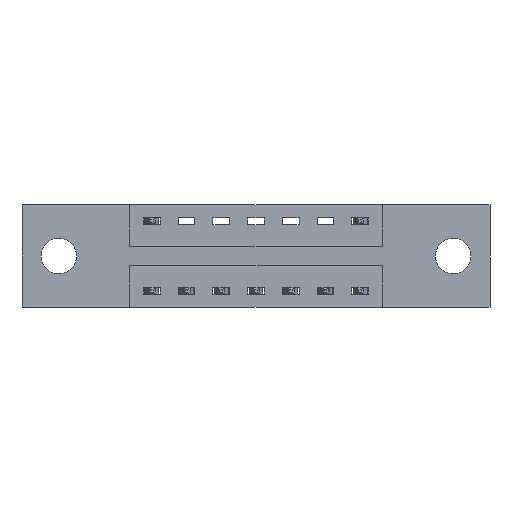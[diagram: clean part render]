
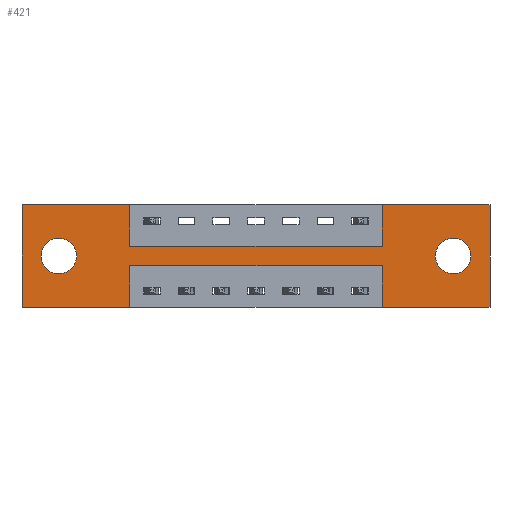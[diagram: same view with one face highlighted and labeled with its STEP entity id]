
A CAD part, front view. The second image highlights one B-rep face of the part: STEP entity #421.
In plain terms, the highlighted planar face has unit normal (0, -1, 0).
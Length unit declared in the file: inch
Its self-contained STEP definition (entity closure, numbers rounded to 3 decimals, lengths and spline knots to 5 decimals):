
#35 = DIRECTION ( 'NONE',  ( -1., 0., 0. ) ) ;
#144 = FACE_BOUND ( 'NONE', #7041, .T. ) ;
#194 = VERTEX_POINT ( 'NONE', #1288 ) ;
#335 = LINE ( 'NONE', #1972, #2369 ) ;
#369 = FACE_BOUND ( 'NONE', #668, .T. ) ;
#400 = CARTESIAN_POINT ( 'NONE',  ( 0.3875, 0., 0. ) ) ;
#421 = ADVANCED_FACE ( 'NONE', ( #144, #369, #7579 ), #6821, .T. ) ;
#471 = VECTOR ( 'NONE', #1988, 39.37008 ) ;
#512 = CARTESIAN_POINT ( 'NONE',  ( 0., 0., 0. ) ) ;
#552 = ORIENTED_EDGE ( 'NONE', *, *, #2028, .F. ) ;
#668 = EDGE_LOOP ( 'NONE', ( #2481, #3615 ) ) ;
#696 = EDGE_CURVE ( 'NONE', #762, #3119, #7354, .T. ) ;
#727 = EDGE_CURVE ( 'NONE', #2300, #6706, #3171, .T. ) ;
#762 = VERTEX_POINT ( 'NONE', #5005 ) ;
#773 = EDGE_CURVE ( 'NONE', #6706, #7704, #6102, .T. ) ;
#774 = EDGE_CURVE ( 'NONE', #7704, #8940, #2515, .T. ) ;
#830 = EDGE_CURVE ( 'NONE', #5140, #2868, #6633, .T. ) ;
#842 = EDGE_CURVE ( 'NONE', #2868, #6374, #4539, .T. ) ;
#863 = VERTEX_POINT ( 'NONE', #1315 ) ;
#911 = EDGE_CURVE ( 'NONE', #6374, #1495, #6934, .T. ) ;
#912 = AXIS2_PLACEMENT_3D ( 'NONE', #7059, #5029, #2269 ) ;
#920 = ORIENTED_EDGE ( 'NONE', *, *, #773, .F. ) ;
#1122 = EDGE_CURVE ( 'NONE', #5067, #194, #6198, .T. ) ;
#1136 = EDGE_CURVE ( 'NONE', #1147, #7518, #8163, .T. ) ;
#1147 = VERTEX_POINT ( 'NONE', #6902 ) ;
#1246 = ORIENTED_EDGE ( 'NONE', *, *, #1746, .F. ) ;
#1274 = AXIS2_PLACEMENT_3D ( 'NONE', #6881, #5798, #4354 ) ;
#1288 = CARTESIAN_POINT ( 'NONE',  ( 0.1325, 0., -0.249 ) ) ;
#1315 = CARTESIAN_POINT ( 'NONE',  ( 0., 0., 0. ) ) ;
#1495 = VERTEX_POINT ( 'NONE', #8687 ) ;
#1498 = EDGE_CURVE ( 'NONE', #1495, #5278, #335, .T. ) ;
#1546 = CARTESIAN_POINT ( 'NONE',  ( 0., 0., 0. ) ) ;
#1619 = CARTESIAN_POINT ( 'NONE',  ( 1.2975, 0., -0.22 ) ) ;
#1699 = VECTOR ( 'NONE', #5994, 39.37008 ) ;
#1746 = EDGE_CURVE ( 'NONE', #3119, #5140, #3695, .T. ) ;
#1870 = DIRECTION ( 'NONE',  ( 0., 1., 0. ) ) ;
#1951 = ORIENTED_EDGE ( 'NONE', *, *, #3240, .T. ) ;
#1972 = CARTESIAN_POINT ( 'NONE',  ( 0., 0., -0.37 ) ) ;
#1988 = DIRECTION ( 'NONE',  ( 1., 0., 0. ) ) ;
#2028 = EDGE_CURVE ( 'NONE', #5278, #863, #4166, .T. ) ;
#2193 = ORIENTED_EDGE ( 'NONE', *, *, #911, .F. ) ;
#2203 = CIRCLE ( 'NONE', #7440, 0.064 ) ;
#2269 = DIRECTION ( 'NONE',  ( 0., 0., -1. ) ) ;
#2300 = VERTEX_POINT ( 'NONE', #400 ) ;
#2369 = VECTOR ( 'NONE', #4577, 39.37008 ) ;
#2481 = ORIENTED_EDGE ( 'NONE', *, *, #1122, .T. ) ;
#2515 = LINE ( 'NONE', #4297, #5889 ) ;
#2553 = ORIENTED_EDGE ( 'NONE', *, *, #830, .F. ) ;
#2560 = CARTESIAN_POINT ( 'NONE',  ( 0., 0., -0.37 ) ) ;
#2620 = LINE ( 'NONE', #8051, #6205 ) ;
#2621 = VECTOR ( 'NONE', #35, 39.37008 ) ;
#2627 = DIRECTION ( 'NONE',  ( 0., 0., 1. ) ) ;
#2783 = DIRECTION ( 'NONE',  ( 0., 1., 0. ) ) ;
#2852 = EDGE_LOOP ( 'NONE', ( #2193, #6976, #2553, #1246, #5279, #5709, #6565, #920, #9067, #6382, #552, #6943 ) ) ;
#2868 = VERTEX_POINT ( 'NONE', #1619 ) ;
#2904 = CARTESIAN_POINT ( 'NONE',  ( 0.3875, 0., -0.37 ) ) ;
#2919 = CARTESIAN_POINT ( 'NONE',  ( 0.3875, 0., -0.22 ) ) ;
#3119 = VERTEX_POINT ( 'NONE', #7501 ) ;
#3131 = EDGE_CURVE ( 'NONE', #194, #5067, #5295, .T. ) ;
#3171 = LINE ( 'NONE', #7918, #6945 ) ;
#3240 = EDGE_CURVE ( 'NONE', #7518, #1147, #2203, .T. ) ;
#3261 = DIRECTION ( 'NONE',  ( 0., 0., -1. ) ) ;
#3263 = EDGE_CURVE ( 'NONE', #863, #2300, #3871, .T. ) ;
#3388 = VECTOR ( 'NONE', #3261, 39.37008 ) ;
#3482 = VECTOR ( 'NONE', #6129, 39.37008 ) ;
#3615 = ORIENTED_EDGE ( 'NONE', *, *, #3131, .T. ) ;
#3630 = DIRECTION ( 'NONE',  ( 0., -1., 0. ) ) ;
#3636 = CARTESIAN_POINT ( 'NONE',  ( 1.2975, 0., -0.15 ) ) ;
#3695 = LINE ( 'NONE', #2560, #3482 ) ;
#3871 = LINE ( 'NONE', #512, #8935 ) ;
#4068 = ORIENTED_EDGE ( 'NONE', *, *, #1136, .T. ) ;
#4108 = DIRECTION ( 'NONE',  ( 0., 0., -1. ) ) ;
#4166 = LINE ( 'NONE', #1546, #6070 ) ;
#4294 = CARTESIAN_POINT ( 'NONE',  ( 0.1325, 0., -0.121 ) ) ;
#4297 = CARTESIAN_POINT ( 'NONE',  ( 1.2975, 0., 0. ) ) ;
#4354 = DIRECTION ( 'NONE',  ( 0., 0., 1. ) ) ;
#4539 = LINE ( 'NONE', #8228, #2621 ) ;
#4577 = DIRECTION ( 'NONE',  ( -1., 0., 0. ) ) ;
#4893 = CARTESIAN_POINT ( 'NONE',  ( 0., 0., -0.37 ) ) ;
#5000 = CARTESIAN_POINT ( 'NONE',  ( 1.5525, 0., -0.249 ) ) ;
#5005 = CARTESIAN_POINT ( 'NONE',  ( 1.685, 0., 0. ) ) ;
#5029 = DIRECTION ( 'NONE',  ( 0., 1., 0. ) ) ;
#5067 = VERTEX_POINT ( 'NONE', #4294 ) ;
#5091 = CARTESIAN_POINT ( 'NONE',  ( 1.685, 0., 0. ) ) ;
#5140 = VERTEX_POINT ( 'NONE', #6533 ) ;
#5170 = AXIS2_PLACEMENT_3D ( 'NONE', #6194, #1870, #6865 ) ;
#5278 = VERTEX_POINT ( 'NONE', #6081 ) ;
#5279 = ORIENTED_EDGE ( 'NONE', *, *, #696, .F. ) ;
#5295 = CIRCLE ( 'NONE', #5170, 0.064 ) ;
#5697 = CARTESIAN_POINT ( 'NONE',  ( 1.2975, 0., -0.37 ) ) ;
#5709 = ORIENTED_EDGE ( 'NONE', *, *, #5861, .F. ) ;
#5798 = DIRECTION ( 'NONE',  ( 0., 1., 0. ) ) ;
#5861 = EDGE_CURVE ( 'NONE', #8940, #762, #2620, .T. ) ;
#5889 = VECTOR ( 'NONE', #2627, 39.37008 ) ;
#5994 = DIRECTION ( 'NONE',  ( 0., 0., -1. ) ) ;
#6070 = VECTOR ( 'NONE', #6574, 39.37008 ) ;
#6081 = CARTESIAN_POINT ( 'NONE',  ( 0., 0., -0.37 ) ) ;
#6102 = LINE ( 'NONE', #7823, #471 ) ;
#6129 = DIRECTION ( 'NONE',  ( -1., 0., 0. ) ) ;
#6194 = CARTESIAN_POINT ( 'NONE',  ( 0.1325, 0., -0.185 ) ) ;
#6198 = CIRCLE ( 'NONE', #1274, 0.064 ) ;
#6205 = VECTOR ( 'NONE', #8079, 39.37008 ) ;
#6374 = VERTEX_POINT ( 'NONE', #2919 ) ;
#6382 = ORIENTED_EDGE ( 'NONE', *, *, #3263, .F. ) ;
#6429 = VECTOR ( 'NONE', #7314, 39.37008 ) ;
#6488 = CARTESIAN_POINT ( 'NONE',  ( 1.2975, 0., 0. ) ) ;
#6533 = CARTESIAN_POINT ( 'NONE',  ( 1.2975, 0., -0.37 ) ) ;
#6565 = ORIENTED_EDGE ( 'NONE', *, *, #774, .F. ) ;
#6574 = DIRECTION ( 'NONE',  ( 0., 0., 1. ) ) ;
#6633 = LINE ( 'NONE', #5697, #6429 ) ;
#6706 = VERTEX_POINT ( 'NONE', #7364 ) ;
#6821 = PLANE ( 'NONE',  #8729 ) ;
#6865 = DIRECTION ( 'NONE',  ( 0., 0., 1. ) ) ;
#6881 = CARTESIAN_POINT ( 'NONE',  ( 0.1325, 0., -0.185 ) ) ;
#6902 = CARTESIAN_POINT ( 'NONE',  ( 1.5525, 0., -0.121 ) ) ;
#6934 = LINE ( 'NONE', #2904, #3388 ) ;
#6943 = ORIENTED_EDGE ( 'NONE', *, *, #1498, .F. ) ;
#6945 = VECTOR ( 'NONE', #7594, 39.37008 ) ;
#6976 = ORIENTED_EDGE ( 'NONE', *, *, #842, .F. ) ;
#7003 = CARTESIAN_POINT ( 'NONE',  ( 1.5525, 0., -0.185 ) ) ;
#7031 = DIRECTION ( 'NONE',  ( 1., 0., 0. ) ) ;
#7041 = EDGE_LOOP ( 'NONE', ( #4068, #1951 ) ) ;
#7059 = CARTESIAN_POINT ( 'NONE',  ( 1.5525, 0., -0.185 ) ) ;
#7314 = DIRECTION ( 'NONE',  ( 0., 0., 1. ) ) ;
#7354 = LINE ( 'NONE', #5091, #1699 ) ;
#7364 = CARTESIAN_POINT ( 'NONE',  ( 0.3875, 0., -0.15 ) ) ;
#7440 = AXIS2_PLACEMENT_3D ( 'NONE', #7003, #2783, #7677 ) ;
#7501 = CARTESIAN_POINT ( 'NONE',  ( 1.685, 0., -0.37 ) ) ;
#7518 = VERTEX_POINT ( 'NONE', #5000 ) ;
#7579 = FACE_OUTER_BOUND ( 'NONE', #2852, .T. ) ;
#7594 = DIRECTION ( 'NONE',  ( 0., 0., -1. ) ) ;
#7677 = DIRECTION ( 'NONE',  ( 0., 0., -1. ) ) ;
#7704 = VERTEX_POINT ( 'NONE', #3636 ) ;
#7823 = CARTESIAN_POINT ( 'NONE',  ( 0.3875, 0., -0.15 ) ) ;
#7918 = CARTESIAN_POINT ( 'NONE',  ( 0.3875, 0., 0. ) ) ;
#8051 = CARTESIAN_POINT ( 'NONE',  ( 0., 0., 0. ) ) ;
#8079 = DIRECTION ( 'NONE',  ( 1., 0., 0. ) ) ;
#8163 = CIRCLE ( 'NONE', #912, 0.064 ) ;
#8228 = CARTESIAN_POINT ( 'NONE',  ( 0.3875, 0., -0.22 ) ) ;
#8687 = CARTESIAN_POINT ( 'NONE',  ( 0.3875, 0., -0.37 ) ) ;
#8729 = AXIS2_PLACEMENT_3D ( 'NONE', #4893, #3630, #4108 ) ;
#8935 = VECTOR ( 'NONE', #7031, 39.37008 ) ;
#8940 = VERTEX_POINT ( 'NONE', #6488 ) ;
#9067 = ORIENTED_EDGE ( 'NONE', *, *, #727, .F. ) ;
